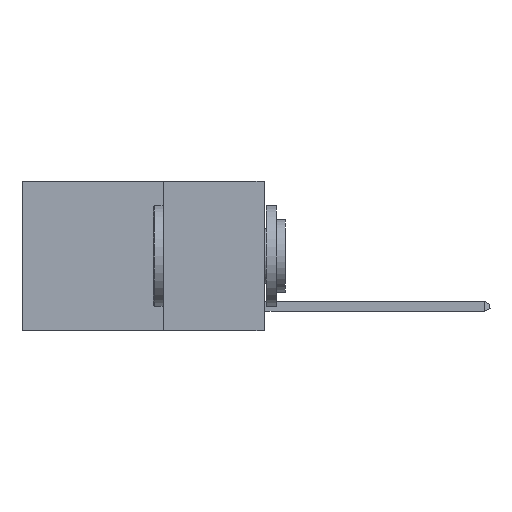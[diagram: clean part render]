
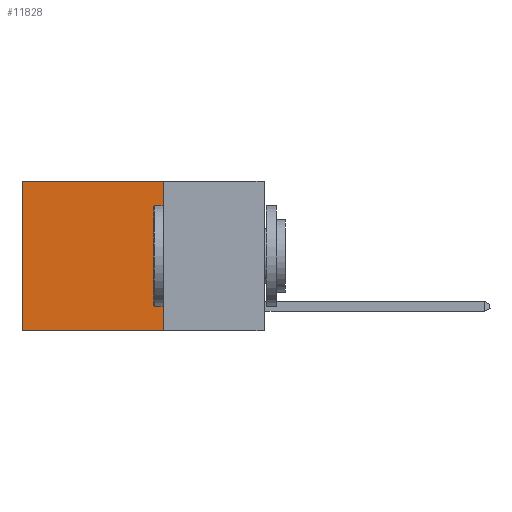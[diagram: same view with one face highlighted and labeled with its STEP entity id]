
A CAD part, left-side view. The second image highlights one B-rep face of the part: STEP entity #11828.
In plain terms, the highlighted planar face has unit normal (-1, 0, 0).
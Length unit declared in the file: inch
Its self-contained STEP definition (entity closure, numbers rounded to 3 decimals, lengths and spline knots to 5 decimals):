
#70 = EDGE_CURVE ( 'NONE', #18951, #7065, #21186, .T. ) ;
#179 = CARTESIAN_POINT ( 'NONE',  ( 0.2625, 0.6, -0.37 ) ) ;
#1474 = VERTEX_POINT ( 'NONE', #13510 ) ;
#1630 = VERTEX_POINT ( 'NONE', #20376 ) ;
#2267 = LINE ( 'NONE', #4013, #15800 ) ;
#2654 = EDGE_CURVE ( 'NONE', #1630, #1474, #2267, .T. ) ;
#4013 = CARTESIAN_POINT ( 'NONE',  ( 0.2625, 0.25, 0. ) ) ;
#5468 = LINE ( 'NONE', #23896, #14410 ) ;
#6735 = AXIS2_PLACEMENT_3D ( 'NONE', #8893, #19070, #7301 ) ;
#7065 = VERTEX_POINT ( 'NONE', #179 ) ;
#7301 = DIRECTION ( 'NONE',  ( 0., 0., -1. ) ) ;
#8893 = CARTESIAN_POINT ( 'NONE',  ( 0.2625, 0.25, 0. ) ) ;
#9153 = VECTOR ( 'NONE', #23320, 39.37008 ) ;
#9846 = DIRECTION ( 'NONE',  ( 0., 1., 0. ) ) ;
#11129 = CARTESIAN_POINT ( 'NONE',  ( 0.2625, 0.6, 0. ) ) ;
#11713 = EDGE_CURVE ( 'NONE', #1630, #18951, #5468, .T. ) ;
#11828 = ADVANCED_FACE ( 'NONE', ( #13003 ), #13135, .F. ) ;
#12323 = CARTESIAN_POINT ( 'NONE',  ( 0.2625, 0.25, -0.37 ) ) ;
#12709 = DIRECTION ( 'NONE',  ( 0., 1., 0. ) ) ;
#13003 = FACE_OUTER_BOUND ( 'NONE', #14013, .T. ) ;
#13121 = ORIENTED_EDGE ( 'NONE', *, *, #22880, .F. ) ;
#13135 = PLANE ( 'NONE',  #6735 ) ;
#13510 = CARTESIAN_POINT ( 'NONE',  ( 0.2625, 0.25, -0.37 ) ) ;
#13889 = VECTOR ( 'NONE', #12709, 39.37008 ) ;
#14013 = EDGE_LOOP ( 'NONE', ( #25749, #13121, #22039, #25278 ) ) ;
#14410 = VECTOR ( 'NONE', #9846, 39.37008 ) ;
#15800 = VECTOR ( 'NONE', #20178, 39.37008 ) ;
#17389 = CARTESIAN_POINT ( 'NONE',  ( 0.2625, 0.6, 0. ) ) ;
#18951 = VERTEX_POINT ( 'NONE', #17389 ) ;
#19070 = DIRECTION ( 'NONE',  ( 1., 0., 0. ) ) ;
#20178 = DIRECTION ( 'NONE',  ( 0., 0., -1. ) ) ;
#20376 = CARTESIAN_POINT ( 'NONE',  ( 0.2625, 0.25, 0. ) ) ;
#21186 = LINE ( 'NONE', #11129, #9153 ) ;
#22039 = ORIENTED_EDGE ( 'NONE', *, *, #2654, .F. ) ;
#22880 = EDGE_CURVE ( 'NONE', #1474, #7065, #24635, .T. ) ;
#23320 = DIRECTION ( 'NONE',  ( 0., 0., -1. ) ) ;
#23896 = CARTESIAN_POINT ( 'NONE',  ( 0.2625, 0.25, 0. ) ) ;
#24635 = LINE ( 'NONE', #12323, #13889 ) ;
#25278 = ORIENTED_EDGE ( 'NONE', *, *, #11713, .T. ) ;
#25749 = ORIENTED_EDGE ( 'NONE', *, *, #70, .T. ) ;
